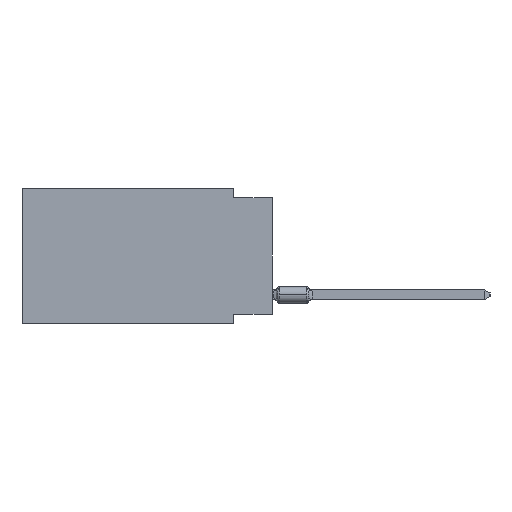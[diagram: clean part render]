
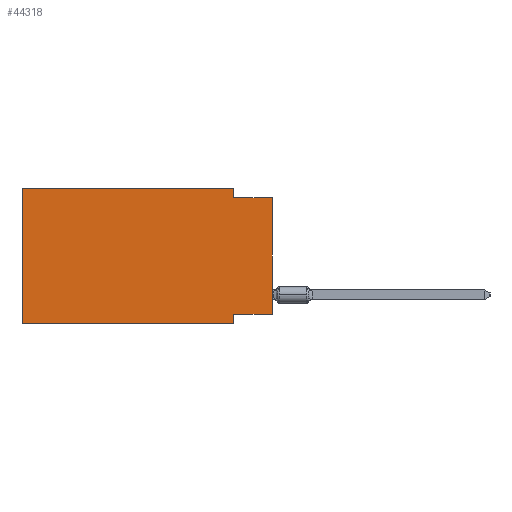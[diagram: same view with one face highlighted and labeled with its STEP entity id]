
A CAD part, left-side view. The second image highlights one B-rep face of the part: STEP entity #44318.
In plain terms, the highlighted planar face has unit normal (-1, 0, 0).
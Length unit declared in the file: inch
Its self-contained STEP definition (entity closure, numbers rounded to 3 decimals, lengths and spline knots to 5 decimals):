
#785 = ORIENTED_EDGE ( 'NONE', *, *, #5026, .F. ) ;
#831 = LINE ( 'NONE', #67934, #46043 ) ;
#3903 = CARTESIAN_POINT ( 'NONE',  ( 0., 0.1, -0.025 ) ) ;
#4478 = EDGE_CURVE ( 'NONE', #35664, #24025, #19365, .T. ) ;
#4819 = CARTESIAN_POINT ( 'NONE',  ( 0., 0.645, -0.35 ) ) ;
#5026 = EDGE_CURVE ( 'NONE', #54772, #35664, #10224, .T. ) ;
#6981 = EDGE_LOOP ( 'NONE', ( #9876, #58016, #785, #42933, #38147, #35286, #27148, #48606 ) ) ;
#7371 = DIRECTION ( 'NONE',  ( 0., 0., -1. ) ) ;
#7635 = DIRECTION ( 'NONE',  ( 0., -1., 0. ) ) ;
#8103 = EDGE_CURVE ( 'NONE', #36703, #58888, #43642, .T. ) ;
#8823 = EDGE_CURVE ( 'NONE', #64024, #27882, #41059, .T. ) ;
#9876 = ORIENTED_EDGE ( 'NONE', *, *, #43068, .T. ) ;
#10224 = LINE ( 'NONE', #47015, #11704 ) ;
#11704 = VECTOR ( 'NONE', #39758, 39.37008 ) ;
#12768 = VECTOR ( 'NONE', #7635, 39.37008 ) ;
#13429 = CARTESIAN_POINT ( 'NONE',  ( 0., 0.645, 0. ) ) ;
#19365 = LINE ( 'NONE', #25856, #12768 ) ;
#20307 = FACE_OUTER_BOUND ( 'NONE', #6981, .T. ) ;
#20716 = VECTOR ( 'NONE', #34019, 39.37008 ) ;
#23628 = EDGE_CURVE ( 'NONE', #64024, #58888, #54498, .T. ) ;
#24025 = VERTEX_POINT ( 'NONE', #78658 ) ;
#24094 = CARTESIAN_POINT ( 'NONE',  ( 0., 0., -0.325 ) ) ;
#25042 = DIRECTION ( 'NONE',  ( 0., 0., -1. ) ) ;
#25856 = CARTESIAN_POINT ( 'NONE',  ( 0., 0., -0.025 ) ) ;
#25899 = LINE ( 'NONE', #69508, #78864 ) ;
#27148 = ORIENTED_EDGE ( 'NONE', *, *, #8103, .F. ) ;
#27882 = VERTEX_POINT ( 'NONE', #73428 ) ;
#29984 = VECTOR ( 'NONE', #25042, 39.37008 ) ;
#31976 = DIRECTION ( 'NONE',  ( 0., 1., 0. ) ) ;
#34019 = DIRECTION ( 'NONE',  ( 0., -1., 0. ) ) ;
#34205 = CARTESIAN_POINT ( 'NONE',  ( 0., 0.1, -0.35 ) ) ;
#35286 = ORIENTED_EDGE ( 'NONE', *, *, #23628, .T. ) ;
#35664 = VERTEX_POINT ( 'NONE', #3903 ) ;
#36703 = VERTEX_POINT ( 'NONE', #38327 ) ;
#38147 = ORIENTED_EDGE ( 'NONE', *, *, #8823, .F. ) ;
#38327 = CARTESIAN_POINT ( 'NONE',  ( 0., 0.1, -0.325 ) ) ;
#38811 = DIRECTION ( 'NONE',  ( 0., 0., 1. ) ) ;
#39758 = DIRECTION ( 'NONE',  ( 0., 0., -1. ) ) ;
#41059 = LINE ( 'NONE', #46723, #75227 ) ;
#42933 = ORIENTED_EDGE ( 'NONE', *, *, #52411, .F. ) ;
#43068 = EDGE_CURVE ( 'NONE', #67481, #24025, #25899, .T. ) ;
#43642 = LINE ( 'NONE', #55774, #29984 ) ;
#44318 = ADVANCED_FACE ( 'NONE', ( #20307 ), #68815, .F. ) ;
#46043 = VECTOR ( 'NONE', #31976, 39.37008 ) ;
#46723 = CARTESIAN_POINT ( 'NONE',  ( 0., 0.645, 0. ) ) ;
#47015 = CARTESIAN_POINT ( 'NONE',  ( 0., 0.1, 0. ) ) ;
#48606 = ORIENTED_EDGE ( 'NONE', *, *, #63773, .F. ) ;
#52411 = EDGE_CURVE ( 'NONE', #27882, #54772, #61148, .T. ) ;
#54105 = DIRECTION ( 'NONE',  ( 0., -1., 0. ) ) ;
#54125 = CARTESIAN_POINT ( 'NONE',  ( 0., 0.1, 0. ) ) ;
#54445 = AXIS2_PLACEMENT_3D ( 'NONE', #13429, #62742, #7371 ) ;
#54498 = LINE ( 'NONE', #59355, #62512 ) ;
#54772 = VERTEX_POINT ( 'NONE', #54125 ) ;
#55774 = CARTESIAN_POINT ( 'NONE',  ( 0., 0.1, -0.35 ) ) ;
#58016 = ORIENTED_EDGE ( 'NONE', *, *, #4478, .F. ) ;
#58888 = VERTEX_POINT ( 'NONE', #34205 ) ;
#59355 = CARTESIAN_POINT ( 'NONE',  ( 0., 0.645, -0.35 ) ) ;
#61148 = LINE ( 'NONE', #79770, #20716 ) ;
#62512 = VECTOR ( 'NONE', #54105, 39.37008 ) ;
#62742 = DIRECTION ( 'NONE',  ( 1., 0., 0. ) ) ;
#63773 = EDGE_CURVE ( 'NONE', #67481, #36703, #831, .T. ) ;
#64024 = VERTEX_POINT ( 'NONE', #4819 ) ;
#66483 = DIRECTION ( 'NONE',  ( 0., 0., 1. ) ) ;
#67481 = VERTEX_POINT ( 'NONE', #24094 ) ;
#67934 = CARTESIAN_POINT ( 'NONE',  ( 0., 0., -0.325 ) ) ;
#68815 = PLANE ( 'NONE',  #54445 ) ;
#69508 = CARTESIAN_POINT ( 'NONE',  ( 0., 0., 0. ) ) ;
#73428 = CARTESIAN_POINT ( 'NONE',  ( 0., 0.645, 0. ) ) ;
#75227 = VECTOR ( 'NONE', #66483, 39.37008 ) ;
#78658 = CARTESIAN_POINT ( 'NONE',  ( 0., 0., -0.025 ) ) ;
#78864 = VECTOR ( 'NONE', #38811, 39.37008 ) ;
#79770 = CARTESIAN_POINT ( 'NONE',  ( 0., 0.645, 0. ) ) ;
